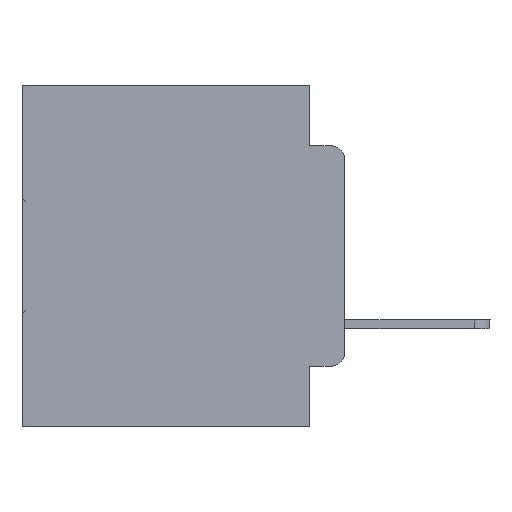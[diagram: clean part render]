
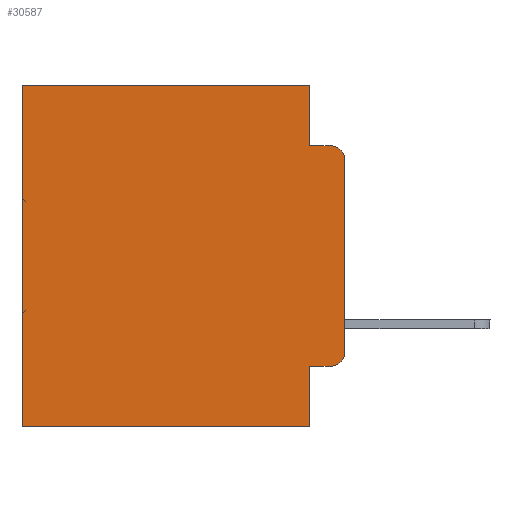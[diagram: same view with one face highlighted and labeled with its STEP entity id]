
A CAD part, left-side view. The second image highlights one B-rep face of the part: STEP entity #30587.
In plain terms, the highlighted planar face has unit normal (-1, 0, 0).
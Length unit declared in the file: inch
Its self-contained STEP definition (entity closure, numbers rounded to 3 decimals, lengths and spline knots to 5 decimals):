
#332 = LINE ( 'NONE', #22955, #21340 ) ;
#455 = AXIS2_PLACEMENT_3D ( 'NONE', #18870, #1291, #21550 ) ;
#667 = DIRECTION ( 'NONE',  ( 0., 0., -1. ) ) ;
#863 = VERTEX_POINT ( 'NONE', #7618 ) ;
#995 = AXIS2_PLACEMENT_3D ( 'NONE', #16066, #18910, #24049 ) ;
#1291 = DIRECTION ( 'NONE',  ( 1., 0., 0. ) ) ;
#1434 = ORIENTED_EDGE ( 'NONE', *, *, #11873, .F. ) ;
#1473 = ORIENTED_EDGE ( 'NONE', *, *, #31507, .F. ) ;
#1715 = CARTESIAN_POINT ( 'NONE',  ( 0.298, 0., 0. ) ) ;
#1825 = DIRECTION ( 'NONE',  ( 0., 1., 0. ) ) ;
#2862 = CARTESIAN_POINT ( 'NONE',  ( 0.298, 0.02, -0.0885 ) ) ;
#3112 = CARTESIAN_POINT ( 'NONE',  ( 0.298, 0.02, -0.1085 ) ) ;
#3150 = EDGE_CURVE ( 'NONE', #26034, #12705, #31263, .T. ) ;
#3337 = LINE ( 'NONE', #13263, #27559 ) ;
#3600 = ORIENTED_EDGE ( 'NONE', *, *, #7946, .T. ) ;
#4367 = VECTOR ( 'NONE', #1825, 39.37008 ) ;
#4457 = DIRECTION ( 'NONE',  ( 0., -1., 0. ) ) ;
#5574 = CARTESIAN_POINT ( 'NONE',  ( 0.298, 0.473, 0. ) ) ;
#5753 = LINE ( 'NONE', #27379, #7376 ) ;
#6065 = VECTOR ( 'NONE', #31101, 39.37008 ) ;
#7376 = VECTOR ( 'NONE', #4457, 39.37008 ) ;
#7615 = VERTEX_POINT ( 'NONE', #2862 ) ;
#7618 = CARTESIAN_POINT ( 'NONE',  ( 0.298, 0., -0.3915 ) ) ;
#7935 = VECTOR ( 'NONE', #14054, 39.37008 ) ;
#7946 = EDGE_CURVE ( 'NONE', #16588, #18760, #5753, .T. ) ;
#8978 = DIRECTION ( 'NONE',  ( 0., 0., -1. ) ) ;
#10825 = DIRECTION ( 'NONE',  ( 0., 0., -1. ) ) ;
#11356 = DIRECTION ( 'NONE',  ( -1., 0., 0. ) ) ;
#11873 = EDGE_CURVE ( 'NONE', #15606, #14653, #16391, .T. ) ;
#12705 = VERTEX_POINT ( 'NONE', #12848 ) ;
#12848 = CARTESIAN_POINT ( 'NONE',  ( 0.298, 0.473, -0.5 ) ) ;
#13086 = EDGE_LOOP ( 'NONE', ( #16865, #27805, #1473, #1434, #20497, #30449, #13763, #18020, #3600, #28992 ) ) ;
#13263 = CARTESIAN_POINT ( 'NONE',  ( 0.298, 0.051, 0. ) ) ;
#13763 = ORIENTED_EDGE ( 'NONE', *, *, #3150, .F. ) ;
#13838 = CARTESIAN_POINT ( 'NONE',  ( 0.298, 0., -0.5 ) ) ;
#14054 = DIRECTION ( 'NONE',  ( 0., 1., 0. ) ) ;
#14653 = VERTEX_POINT ( 'NONE', #26951 ) ;
#14780 = LINE ( 'NONE', #5574, #30996 ) ;
#15286 = CIRCLE ( 'NONE', #995, 0.02 ) ;
#15564 = EDGE_CURVE ( 'NONE', #17559, #7615, #29560, .T. ) ;
#15606 = VERTEX_POINT ( 'NONE', #21599 ) ;
#15696 = EDGE_CURVE ( 'NONE', #18760, #863, #15286, .T. ) ;
#15742 = EDGE_CURVE ( 'NONE', #17559, #863, #17268, .T. ) ;
#16066 = CARTESIAN_POINT ( 'NONE',  ( 0.298, 0.02, -0.3915 ) ) ;
#16082 = CARTESIAN_POINT ( 'NONE',  ( 0.298, 0.051, 0. ) ) ;
#16370 = PLANE ( 'NONE',  #455 ) ;
#16391 = LINE ( 'NONE', #16082, #6065 ) ;
#16435 = DIRECTION ( 'NONE',  ( 0., 0., -1. ) ) ;
#16588 = VERTEX_POINT ( 'NONE', #31607 ) ;
#16865 = ORIENTED_EDGE ( 'NONE', *, *, #15742, .F. ) ;
#17011 = CARTESIAN_POINT ( 'NONE',  ( 0.298, 0., -0.1085 ) ) ;
#17268 = LINE ( 'NONE', #31213, #25587 ) ;
#17559 = VERTEX_POINT ( 'NONE', #17011 ) ;
#18020 = ORIENTED_EDGE ( 'NONE', *, *, #23867, .F. ) ;
#18760 = VERTEX_POINT ( 'NONE', #21583 ) ;
#18870 = CARTESIAN_POINT ( 'NONE',  ( 0.298, 0., 0. ) ) ;
#18910 = DIRECTION ( 'NONE',  ( -1., 0., 0. ) ) ;
#20013 = CARTESIAN_POINT ( 'NONE',  ( 0.298, 0.051, -0.5 ) ) ;
#20497 = ORIENTED_EDGE ( 'NONE', *, *, #26678, .T. ) ;
#20543 = CARTESIAN_POINT ( 'NONE',  ( 0.298, 0.473, 0. ) ) ;
#21340 = VECTOR ( 'NONE', #25503, 39.37008 ) ;
#21550 = DIRECTION ( 'NONE',  ( 0., 0., -1. ) ) ;
#21583 = CARTESIAN_POINT ( 'NONE',  ( 0.298, 0.02, -0.4115 ) ) ;
#21599 = CARTESIAN_POINT ( 'NONE',  ( 0.298, 0.051, 0. ) ) ;
#22955 = CARTESIAN_POINT ( 'NONE',  ( 0.298, 0.051, -0.0885 ) ) ;
#23867 = EDGE_CURVE ( 'NONE', #16588, #26034, #3337, .T. ) ;
#24049 = DIRECTION ( 'NONE',  ( 0., 0., -1. ) ) ;
#25072 = EDGE_CURVE ( 'NONE', #32180, #12705, #14780, .T. ) ;
#25503 = DIRECTION ( 'NONE',  ( 0., -1., 0. ) ) ;
#25587 = VECTOR ( 'NONE', #16435, 39.37008 ) ;
#26034 = VERTEX_POINT ( 'NONE', #20013 ) ;
#26678 = EDGE_CURVE ( 'NONE', #15606, #32180, #31694, .T. ) ;
#26951 = CARTESIAN_POINT ( 'NONE',  ( 0.298, 0.051, -0.0885 ) ) ;
#27379 = CARTESIAN_POINT ( 'NONE',  ( 0.298, 0.051, -0.4115 ) ) ;
#27559 = VECTOR ( 'NONE', #10825, 39.37008 ) ;
#27805 = ORIENTED_EDGE ( 'NONE', *, *, #15564, .T. ) ;
#28991 = AXIS2_PLACEMENT_3D ( 'NONE', #3112, #11356, #8978 ) ;
#28992 = ORIENTED_EDGE ( 'NONE', *, *, #15696, .T. ) ;
#29560 = CIRCLE ( 'NONE', #28991, 0.02 ) ;
#30449 = ORIENTED_EDGE ( 'NONE', *, *, #25072, .T. ) ;
#30587 = ADVANCED_FACE ( 'NONE', ( #32508 ), #16370, .F. ) ;
#30996 = VECTOR ( 'NONE', #667, 39.37008 ) ;
#31101 = DIRECTION ( 'NONE',  ( 0., 0., -1. ) ) ;
#31213 = CARTESIAN_POINT ( 'NONE',  ( 0.298, 0., 0. ) ) ;
#31263 = LINE ( 'NONE', #13838, #7935 ) ;
#31507 = EDGE_CURVE ( 'NONE', #14653, #7615, #332, .T. ) ;
#31607 = CARTESIAN_POINT ( 'NONE',  ( 0.298, 0.051, -0.4115 ) ) ;
#31694 = LINE ( 'NONE', #1715, #4367 ) ;
#32180 = VERTEX_POINT ( 'NONE', #20543 ) ;
#32508 = FACE_OUTER_BOUND ( 'NONE', #13086, .T. ) ;
